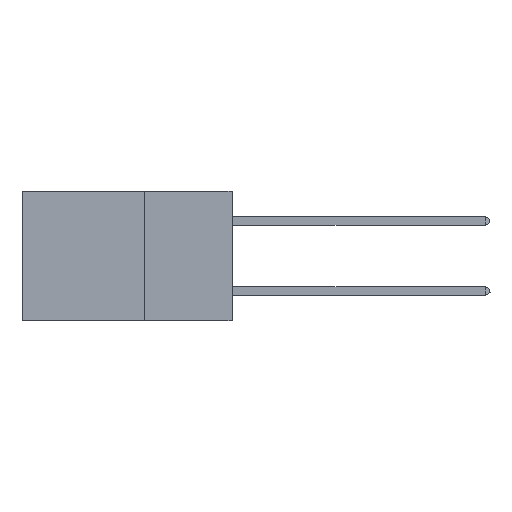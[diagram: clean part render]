
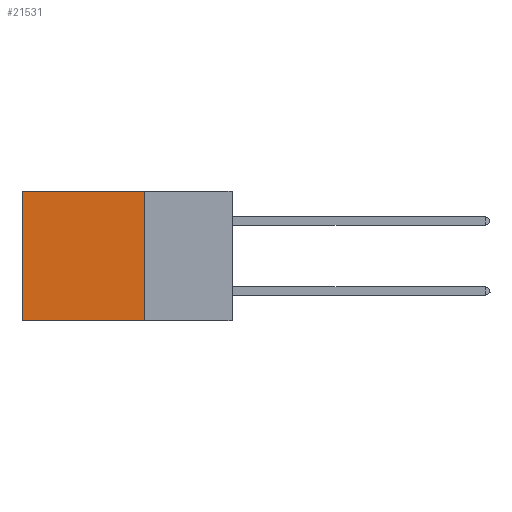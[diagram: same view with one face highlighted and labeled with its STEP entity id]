
A CAD part, left-side view. The second image highlights one B-rep face of the part: STEP entity #21531.
In plain terms, the highlighted planar face has unit normal (-1, 0, 0).
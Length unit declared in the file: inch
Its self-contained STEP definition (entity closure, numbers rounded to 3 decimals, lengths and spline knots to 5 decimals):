
#145 = AXIS2_PLACEMENT_3D ( 'NONE', #37852, #4291, #13981 ) ;
#209 = CARTESIAN_POINT ( 'NONE',  ( 0.2875, 0.25, 0. ) ) ;
#699 = VERTEX_POINT ( 'NONE', #36731 ) ;
#1763 = PLANE ( 'NONE',  #145 ) ;
#2198 = CARTESIAN_POINT ( 'NONE',  ( 0.2875, 0.6, 0. ) ) ;
#3921 = EDGE_CURVE ( 'NONE', #699, #36160, #17456, .T. ) ;
#4291 = DIRECTION ( 'NONE',  ( 1., 0., 0. ) ) ;
#4330 = LINE ( 'NONE', #26986, #29063 ) ;
#7182 = VERTEX_POINT ( 'NONE', #2198 ) ;
#8520 = VECTOR ( 'NONE', #36027, 39.37008 ) ;
#9168 = DIRECTION ( 'NONE',  ( 0., 0., -1. ) ) ;
#12422 = CARTESIAN_POINT ( 'NONE',  ( 0.2875, 0.25, 0. ) ) ;
#12617 = VECTOR ( 'NONE', #15630, 39.37008 ) ;
#13789 = CARTESIAN_POINT ( 'NONE',  ( 0.2875, 0.6, -0.37 ) ) ;
#13981 = DIRECTION ( 'NONE',  ( 0., 0., -1. ) ) ;
#15012 = ORIENTED_EDGE ( 'NONE', *, *, #21891, .T. ) ;
#15216 = ORIENTED_EDGE ( 'NONE', *, *, #27000, .T. ) ;
#15630 = DIRECTION ( 'NONE',  ( 0., 0., -1. ) ) ;
#16520 = VECTOR ( 'NONE', #26579, 39.37008 ) ;
#16622 = LINE ( 'NONE', #12422, #8520 ) ;
#17456 = LINE ( 'NONE', #23390, #16520 ) ;
#20699 = LINE ( 'NONE', #209, #12617 ) ;
#21531 = ADVANCED_FACE ( 'NONE', ( #22921 ), #1763, .F. ) ;
#21631 = ORIENTED_EDGE ( 'NONE', *, *, #34617, .F. ) ;
#21891 = EDGE_CURVE ( 'NONE', #7182, #36160, #4330, .T. ) ;
#22921 = FACE_OUTER_BOUND ( 'NONE', #34975, .T. ) ;
#23390 = CARTESIAN_POINT ( 'NONE',  ( 0.2875, 0.25, -0.37 ) ) ;
#26579 = DIRECTION ( 'NONE',  ( 0., 1., 0. ) ) ;
#26986 = CARTESIAN_POINT ( 'NONE',  ( 0.2875, 0.6, 0. ) ) ;
#27000 = EDGE_CURVE ( 'NONE', #31716, #7182, #16622, .T. ) ;
#29063 = VECTOR ( 'NONE', #9168, 39.37008 ) ;
#29367 = CARTESIAN_POINT ( 'NONE',  ( 0.2875, 0.25, 0. ) ) ;
#31716 = VERTEX_POINT ( 'NONE', #29367 ) ;
#34617 = EDGE_CURVE ( 'NONE', #31716, #699, #20699, .T. ) ;
#34923 = ORIENTED_EDGE ( 'NONE', *, *, #3921, .F. ) ;
#34975 = EDGE_LOOP ( 'NONE', ( #15012, #34923, #21631, #15216 ) ) ;
#36027 = DIRECTION ( 'NONE',  ( 0., 1., 0. ) ) ;
#36160 = VERTEX_POINT ( 'NONE', #13789 ) ;
#36731 = CARTESIAN_POINT ( 'NONE',  ( 0.2875, 0.25, -0.37 ) ) ;
#37852 = CARTESIAN_POINT ( 'NONE',  ( 0.2875, 0.25, 0. ) ) ;
